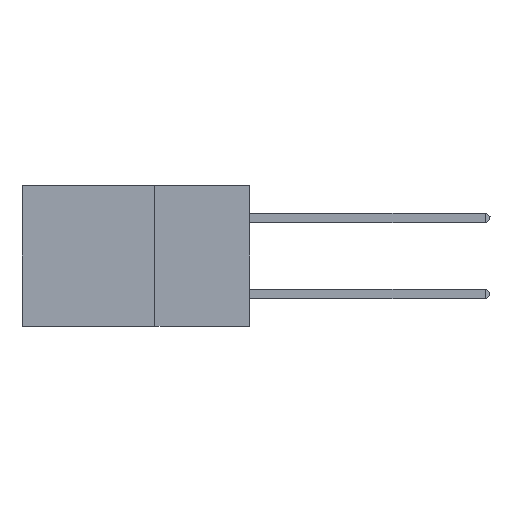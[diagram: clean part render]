
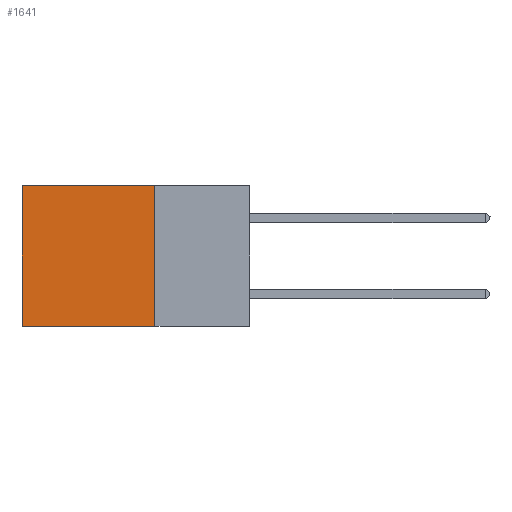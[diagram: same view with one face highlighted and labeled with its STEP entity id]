
A CAD part, left-side view. The second image highlights one B-rep face of the part: STEP entity #1641.
In plain terms, the highlighted planar face has unit normal (-1, 0, 0).
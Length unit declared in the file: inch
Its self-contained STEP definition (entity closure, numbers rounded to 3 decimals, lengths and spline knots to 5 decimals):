
#697 = CARTESIAN_POINT ( 'NONE',  ( 0.2875, 0.6, 0. ) ) ;
#812 = ORIENTED_EDGE ( 'NONE', *, *, #24203, .F. ) ;
#1593 = DIRECTION ( 'NONE',  ( 0., 0., -1. ) ) ;
#1641 = ADVANCED_FACE ( 'NONE', ( #17384 ), #11008, .F. ) ;
#2568 = DIRECTION ( 'NONE',  ( 0., 0., -1. ) ) ;
#3591 = VECTOR ( 'NONE', #13147, 39.37008 ) ;
#3811 = AXIS2_PLACEMENT_3D ( 'NONE', #8970, #25718, #2568 ) ;
#4209 = DIRECTION ( 'NONE',  ( 0., 1., 0. ) ) ;
#4394 = ORIENTED_EDGE ( 'NONE', *, *, #19483, .F. ) ;
#5091 = VECTOR ( 'NONE', #1593, 39.37008 ) ;
#5214 = CARTESIAN_POINT ( 'NONE',  ( 0.2875, 0.25, 0. ) ) ;
#5958 = CARTESIAN_POINT ( 'NONE',  ( 0.2875, 0.25, 0. ) ) ;
#6250 = LINE ( 'NONE', #14567, #10441 ) ;
#6772 = VECTOR ( 'NONE', #25893, 39.37008 ) ;
#7612 = EDGE_CURVE ( 'NONE', #13942, #25040, #15184, .T. ) ;
#7722 = LINE ( 'NONE', #5958, #5091 ) ;
#8970 = CARTESIAN_POINT ( 'NONE',  ( 0.2875, 0.25, 0. ) ) ;
#9144 = LINE ( 'NONE', #697, #6772 ) ;
#9962 = CARTESIAN_POINT ( 'NONE',  ( 0.2875, 0.6, 0. ) ) ;
#10441 = VECTOR ( 'NONE', #4209, 39.37008 ) ;
#10823 = CARTESIAN_POINT ( 'NONE',  ( 0.2875, 0.6, -0.37 ) ) ;
#11008 = PLANE ( 'NONE',  #3811 ) ;
#11200 = CARTESIAN_POINT ( 'NONE',  ( 0.2875, 0.25, -0.37 ) ) ;
#13147 = DIRECTION ( 'NONE',  ( 0., 1., 0. ) ) ;
#13570 = ORIENTED_EDGE ( 'NONE', *, *, #17708, .T. ) ;
#13942 = VERTEX_POINT ( 'NONE', #17418 ) ;
#14567 = CARTESIAN_POINT ( 'NONE',  ( 0.2875, 0.25, -0.37 ) ) ;
#14761 = ORIENTED_EDGE ( 'NONE', *, *, #7612, .T. ) ;
#15184 = LINE ( 'NONE', #5214, #3591 ) ;
#15508 = EDGE_LOOP ( 'NONE', ( #13570, #812, #4394, #14761 ) ) ;
#15701 = VERTEX_POINT ( 'NONE', #10823 ) ;
#15847 = VERTEX_POINT ( 'NONE', #11200 ) ;
#17384 = FACE_OUTER_BOUND ( 'NONE', #15508, .T. ) ;
#17418 = CARTESIAN_POINT ( 'NONE',  ( 0.2875, 0.25, 0. ) ) ;
#17708 = EDGE_CURVE ( 'NONE', #25040, #15701, #9144, .T. ) ;
#19483 = EDGE_CURVE ( 'NONE', #13942, #15847, #7722, .T. ) ;
#24203 = EDGE_CURVE ( 'NONE', #15847, #15701, #6250, .T. ) ;
#25040 = VERTEX_POINT ( 'NONE', #9962 ) ;
#25718 = DIRECTION ( 'NONE',  ( 1., 0., 0. ) ) ;
#25893 = DIRECTION ( 'NONE',  ( 0., 0., -1. ) ) ;
